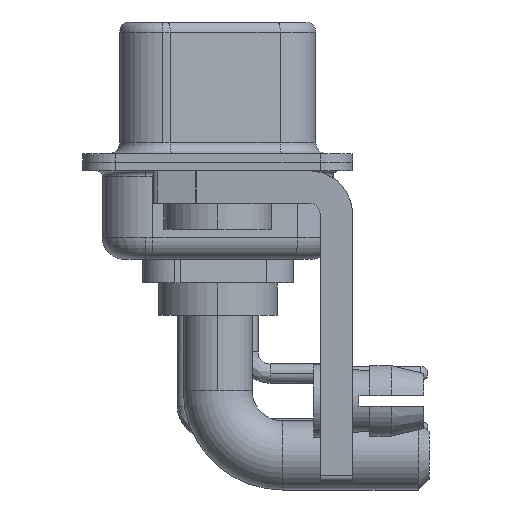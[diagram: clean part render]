
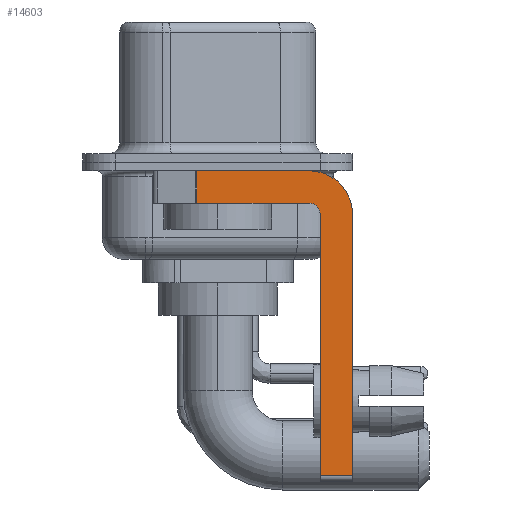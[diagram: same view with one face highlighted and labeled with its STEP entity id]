
A CAD part, left-side view. The second image highlights one B-rep face of the part: STEP entity #14603.
In plain terms, the highlighted planar face has unit normal (-1, 0, 0).
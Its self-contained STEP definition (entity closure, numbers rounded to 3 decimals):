
#95 = VECTOR ( 'NONE', #22716, 1000. ) ;
#406 = DIRECTION ( 'NONE',  ( 0., -1., 0. ) ) ;
#1284 = LINE ( 'NONE', #18617, #95 ) ;
#1943 = VERTEX_POINT ( 'NONE', #24758 ) ;
#1976 = CIRCLE ( 'NONE', #27110, 0.5 ) ;
#2906 = VECTOR ( 'NONE', #15735, 1000. ) ;
#3746 = CARTESIAN_POINT ( 'NONE',  ( -2.9, -4.25, -2.4 ) ) ;
#3867 = EDGE_CURVE ( 'NONE', #6912, #21965, #16107, .T. ) ;
#4050 = CARTESIAN_POINT ( 'NONE',  ( -2.9, -4.75, -2.4 ) ) ;
#4248 = CARTESIAN_POINT ( 'NONE',  ( -2.9, -4.25, -0.4 ) ) ;
#4978 = EDGE_CURVE ( 'NONE', #22546, #6912, #13284, .T. ) ;
#5697 = DIRECTION ( 'NONE',  ( 1., 0., 0. ) ) ;
#6034 = LINE ( 'NONE', #16683, #27303 ) ;
#6615 = ORIENTED_EDGE ( 'NONE', *, *, #21374, .T. ) ;
#6688 = CARTESIAN_POINT ( 'NONE',  ( -2.9, 0.978, -0.4 ) ) ;
#6820 = CARTESIAN_POINT ( 'NONE',  ( -2.9, -4.75, -14.55 ) ) ;
#6852 = ORIENTED_EDGE ( 'NONE', *, *, #10303, .F. ) ;
#6912 = VERTEX_POINT ( 'NONE', #4248 ) ;
#7345 = VERTEX_POINT ( 'NONE', #6820 ) ;
#8265 = VECTOR ( 'NONE', #18026, 1000. ) ;
#8414 = EDGE_CURVE ( 'NONE', #21965, #9942, #6034, .T. ) ;
#8822 = VERTEX_POINT ( 'NONE', #4050 ) ;
#9460 = LINE ( 'NONE', #16266, #25526 ) ;
#9561 = LINE ( 'NONE', #22412, #8265 ) ;
#9942 = VERTEX_POINT ( 'NONE', #25247 ) ;
#10303 = EDGE_CURVE ( 'NONE', #8822, #27222, #1976, .T. ) ;
#10373 = AXIS2_PLACEMENT_3D ( 'NONE', #12671, #25354, #21360 ) ;
#12123 = ORIENTED_EDGE ( 'NONE', *, *, #4978, .F. ) ;
#12390 = CARTESIAN_POINT ( 'NONE',  ( -2.9, -4.25, -2.4 ) ) ;
#12671 = CARTESIAN_POINT ( 'NONE',  ( -2.9, -4.25, -2.4 ) ) ;
#13284 = LINE ( 'NONE', #14950, #13428 ) ;
#13428 = VECTOR ( 'NONE', #406, 1000. ) ;
#13476 = EDGE_LOOP ( 'NONE', ( #12123, #6615, #16913, #6852, #19481, #18306, #14596, #23085 ) ) ;
#13760 = DIRECTION ( 'NONE',  ( 0., -1., 0. ) ) ;
#14176 = CARTESIAN_POINT ( 'NONE',  ( -2.9, -6.25, -2.4 ) ) ;
#14596 = ORIENTED_EDGE ( 'NONE', *, *, #8414, .F. ) ;
#14603 = ADVANCED_FACE ( 'NONE', ( #16213 ), #24604, .F. ) ;
#14950 = CARTESIAN_POINT ( 'NONE',  ( -2.9, 3., -0.4 ) ) ;
#15602 = CARTESIAN_POINT ( 'NONE',  ( -2.9, 0.978, -1.9 ) ) ;
#15735 = DIRECTION ( 'NONE',  ( 0., 0., -1. ) ) ;
#16107 = CIRCLE ( 'NONE', #10373, 2. ) ;
#16213 = FACE_OUTER_BOUND ( 'NONE', #13476, .T. ) ;
#16266 = CARTESIAN_POINT ( 'NONE',  ( -2.9, -4.25, -14.55 ) ) ;
#16683 = CARTESIAN_POINT ( 'NONE',  ( -2.9, -6.25, -2.4 ) ) ;
#16913 = ORIENTED_EDGE ( 'NONE', *, *, #22590, .F. ) ;
#17664 = EDGE_CURVE ( 'NONE', #7345, #9942, #9460, .T. ) ;
#18026 = DIRECTION ( 'NONE',  ( 0., 1., 0. ) ) ;
#18306 = ORIENTED_EDGE ( 'NONE', *, *, #17664, .T. ) ;
#18617 = CARTESIAN_POINT ( 'NONE',  ( -2.9, -4.75, -14.8 ) ) ;
#19481 = ORIENTED_EDGE ( 'NONE', *, *, #20523, .F. ) ;
#20153 = LINE ( 'NONE', #15602, #2906 ) ;
#20523 = EDGE_CURVE ( 'NONE', #7345, #8822, #1284, .T. ) ;
#20678 = DIRECTION ( 'NONE',  ( 0., 0., -1. ) ) ;
#21360 = DIRECTION ( 'NONE',  ( 0., 0., -1. ) ) ;
#21374 = EDGE_CURVE ( 'NONE', #22546, #1943, #20153, .T. ) ;
#21965 = VERTEX_POINT ( 'NONE', #14176 ) ;
#22412 = CARTESIAN_POINT ( 'NONE',  ( -2.9, -4.25, -1.9 ) ) ;
#22544 = DIRECTION ( 'NONE',  ( 0., 0., -1. ) ) ;
#22546 = VERTEX_POINT ( 'NONE', #6688 ) ;
#22590 = EDGE_CURVE ( 'NONE', #27222, #1943, #9561, .T. ) ;
#22716 = DIRECTION ( 'NONE',  ( 0., 0., 1. ) ) ;
#23085 = ORIENTED_EDGE ( 'NONE', *, *, #3867, .F. ) ;
#24590 = AXIS2_PLACEMENT_3D ( 'NONE', #3746, #5697, #22544 ) ;
#24604 = PLANE ( 'NONE',  #24590 ) ;
#24758 = CARTESIAN_POINT ( 'NONE',  ( -2.9, 0.978, -1.9 ) ) ;
#24943 = DIRECTION ( 'NONE',  ( -1., 0., 0. ) ) ;
#25247 = CARTESIAN_POINT ( 'NONE',  ( -2.9, -6.25, -14.55 ) ) ;
#25280 = CARTESIAN_POINT ( 'NONE',  ( -2.9, -4.25, -1.9 ) ) ;
#25354 = DIRECTION ( 'NONE',  ( 1., 0., 0. ) ) ;
#25526 = VECTOR ( 'NONE', #13760, 1000. ) ;
#25700 = DIRECTION ( 'NONE',  ( 0., 0., 1. ) ) ;
#27110 = AXIS2_PLACEMENT_3D ( 'NONE', #12390, #24943, #25700 ) ;
#27222 = VERTEX_POINT ( 'NONE', #25280 ) ;
#27303 = VECTOR ( 'NONE', #20678, 1000. ) ;
